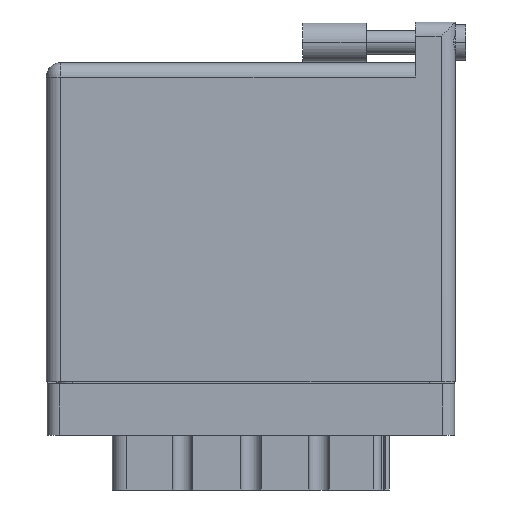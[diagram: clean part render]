
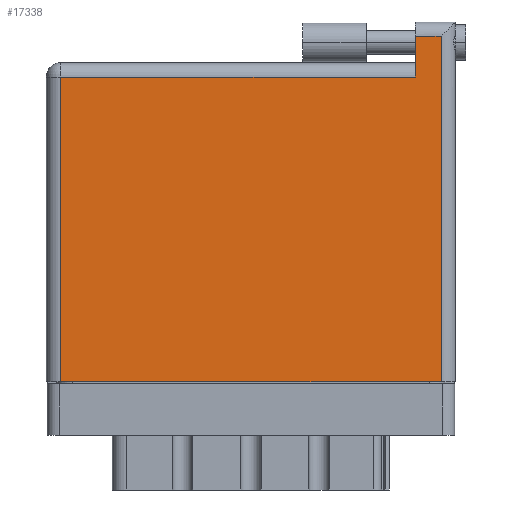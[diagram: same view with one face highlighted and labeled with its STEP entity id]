
A CAD part, front view. The second image highlights one B-rep face of the part: STEP entity #17338.
In plain terms, the highlighted face is planar.
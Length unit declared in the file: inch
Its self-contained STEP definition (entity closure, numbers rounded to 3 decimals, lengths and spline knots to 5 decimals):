
#2528 = VERTEX_POINT ( 'NONE', #6640 ) ;
#2731 = CARTESIAN_POINT ( 'NONE',  ( 0., 1.496, 0. ) ) ;
#3179 = ORIENTED_EDGE ( 'NONE', *, *, #6620, .T. ) ;
#3384 = CARTESIAN_POINT ( 'NONE',  ( 1.938, 0., 0. ) ) ;
#3453 = ORIENTED_EDGE ( 'NONE', *, *, #25305, .T. ) ;
#3615 = CARTESIAN_POINT ( 'NONE',  ( 1.811, 1.696, 0. ) ) ;
#3866 = VERTEX_POINT ( 'NONE', #31686 ) ;
#4789 = VERTEX_POINT ( 'NONE', #3384 ) ;
#4845 = VERTEX_POINT ( 'NONE', #3615 ) ;
#5342 = EDGE_CURVE ( 'NONE', #4789, #2528, #29287, .T. ) ;
#5471 = CARTESIAN_POINT ( 'NONE',  ( 0.07, 0., 0. ) ) ;
#6620 = EDGE_CURVE ( 'NONE', #3866, #4789, #30452, .T. ) ;
#6640 = CARTESIAN_POINT ( 'NONE',  ( 1.938, 1.696, 0. ) ) ;
#6777 = CARTESIAN_POINT ( 'NONE',  ( 0.07, 1.496, 0. ) ) ;
#7891 = VERTEX_POINT ( 'NONE', #24827 ) ;
#8102 = EDGE_CURVE ( 'NONE', #2528, #4845, #15067, .T. ) ;
#8413 = EDGE_CURVE ( 'NONE', #4845, #7891, #9003, .T. ) ;
#8887 = FACE_OUTER_BOUND ( 'NONE', #12852, .T. ) ;
#9003 = LINE ( 'NONE', #12547, #26123 ) ;
#9274 = DIRECTION ( 'NONE',  ( 0., 0., -1. ) ) ;
#9917 = CARTESIAN_POINT ( 'NONE',  ( 0., 0., 0. ) ) ;
#10266 = VECTOR ( 'NONE', #31020, 39.37008 ) ;
#11005 = VECTOR ( 'NONE', #20412, 39.37008 ) ;
#12303 = ORIENTED_EDGE ( 'NONE', *, *, #8102, .T. ) ;
#12547 = CARTESIAN_POINT ( 'NONE',  ( 1.811, 1.766, 0. ) ) ;
#12852 = EDGE_LOOP ( 'NONE', ( #3179, #32408, #12303, #28261, #3453, #30723 ) ) ;
#13360 = CARTESIAN_POINT ( 'NONE',  ( 0., 1.696, 0. ) ) ;
#15067 = LINE ( 'NONE', #13360, #10266 ) ;
#16979 = DIRECTION ( 'NONE',  ( 0., 1., 0. ) ) ;
#17066 = CARTESIAN_POINT ( 'NONE',  ( 0., 1.566, 0. ) ) ;
#17338 = ADVANCED_FACE ( 'NONE', ( #8887 ), #19949, .F. ) ;
#17401 = DIRECTION ( 'NONE',  ( -1., 0., 0. ) ) ;
#19949 = PLANE ( 'NONE',  #31928 ) ;
#19986 = DIRECTION ( 'NONE',  ( 0., -1., 0. ) ) ;
#20032 = VECTOR ( 'NONE', #30982, 39.37008 ) ;
#20412 = DIRECTION ( 'NONE',  ( -1., 0., 0. ) ) ;
#20937 = VECTOR ( 'NONE', #32373, 39.37008 ) ;
#23566 = CARTESIAN_POINT ( 'NONE',  ( 1.938, 1.766, 0. ) ) ;
#24537 = LINE ( 'NONE', #2731, #11005 ) ;
#24827 = CARTESIAN_POINT ( 'NONE',  ( 1.811, 1.496, 0. ) ) ;
#24935 = VECTOR ( 'NONE', #16979, 39.37008 ) ;
#25305 = EDGE_CURVE ( 'NONE', #7891, #27131, #24537, .T. ) ;
#26123 = VECTOR ( 'NONE', #19986, 39.37008 ) ;
#26800 = LINE ( 'NONE', #5471, #20032 ) ;
#27131 = VERTEX_POINT ( 'NONE', #6777 ) ;
#28261 = ORIENTED_EDGE ( 'NONE', *, *, #8413, .T. ) ;
#29287 = LINE ( 'NONE', #23566, #24935 ) ;
#30202 = EDGE_CURVE ( 'NONE', #27131, #3866, #26800, .T. ) ;
#30452 = LINE ( 'NONE', #9917, #20937 ) ;
#30723 = ORIENTED_EDGE ( 'NONE', *, *, #30202, .T. ) ;
#30982 = DIRECTION ( 'NONE',  ( 0., -1., 0. ) ) ;
#31020 = DIRECTION ( 'NONE',  ( -1., 0., 0. ) ) ;
#31686 = CARTESIAN_POINT ( 'NONE',  ( 0.07, 0., 0. ) ) ;
#31928 = AXIS2_PLACEMENT_3D ( 'NONE', #17066, #9274, #17401 ) ;
#32373 = DIRECTION ( 'NONE',  ( 1., 0., 0. ) ) ;
#32408 = ORIENTED_EDGE ( 'NONE', *, *, #5342, .T. ) ;
